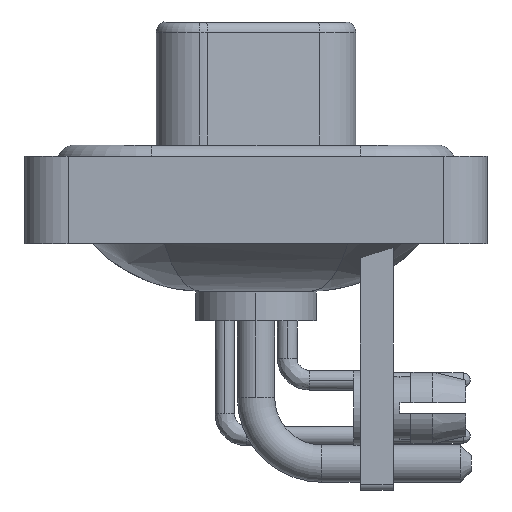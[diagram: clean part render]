
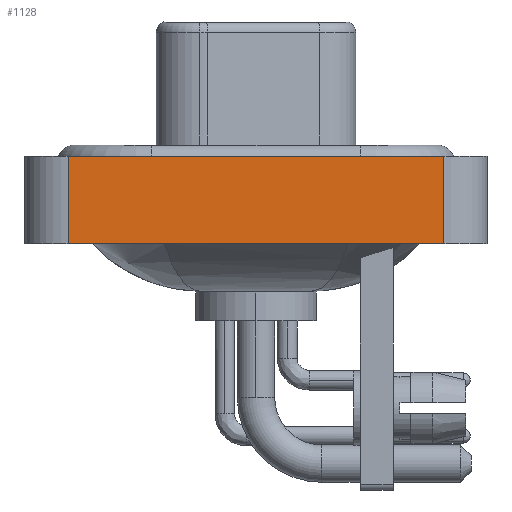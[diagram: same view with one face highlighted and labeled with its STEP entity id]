
A CAD part, left-side view. The second image highlights one B-rep face of the part: STEP entity #1128.
In plain terms, the highlighted planar face has unit normal (-1, 0, 0).
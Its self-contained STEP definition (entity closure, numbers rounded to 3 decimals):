
#1128 = ADVANCED_FACE ( 'NONE', ( #11209 ), #13248, .T. ) ;
#1898 = CARTESIAN_POINT ( 'NONE',  ( -7.3, -8.55, -3.6 ) ) ;
#1907 = DIRECTION ( 'NONE',  ( 0., -1., 0. ) ) ;
#2004 = LINE ( 'NONE', #8308, #26849 ) ;
#3120 = CARTESIAN_POINT ( 'NONE',  ( -7.3, 8.55, -3.6 ) ) ;
#3679 = VERTEX_POINT ( 'NONE', #11744 ) ;
#3937 = DIRECTION ( 'NONE',  ( 0., 0., 1. ) ) ;
#4136 = EDGE_CURVE ( 'NONE', #19035, #3679, #15676, .T. ) ;
#4199 = ORIENTED_EDGE ( 'NONE', *, *, #4136, .F. ) ;
#5425 = VERTEX_POINT ( 'NONE', #26223 ) ;
#7392 = VECTOR ( 'NONE', #19734, 1000. ) ;
#8188 = AXIS2_PLACEMENT_3D ( 'NONE', #15443, #19654, #15731 ) ;
#8308 = CARTESIAN_POINT ( 'NONE',  ( -7.3, -8.55, 0.4 ) ) ;
#8679 = VECTOR ( 'NONE', #16753, 1000. ) ;
#10782 = ORIENTED_EDGE ( 'NONE', *, *, #14921, .T. ) ;
#11209 = FACE_OUTER_BOUND ( 'NONE', #12817, .T. ) ;
#11744 = CARTESIAN_POINT ( 'NONE',  ( -7.3, 8.55, 0.4 ) ) ;
#12044 = EDGE_CURVE ( 'NONE', #19035, #5425, #12382, .T. ) ;
#12382 = LINE ( 'NONE', #1898, #8679 ) ;
#12817 = EDGE_LOOP ( 'NONE', ( #10782, #26274, #4199, #24567 ) ) ;
#13248 = PLANE ( 'NONE',  #8188 ) ;
#14921 = EDGE_CURVE ( 'NONE', #5425, #16706, #25153, .T. ) ;
#15443 = CARTESIAN_POINT ( 'NONE',  ( -7.3, -8.55, -3.6 ) ) ;
#15676 = LINE ( 'NONE', #3120, #7392 ) ;
#15731 = DIRECTION ( 'NONE',  ( 0., 0., 1. ) ) ;
#16704 = CARTESIAN_POINT ( 'NONE',  ( -7.3, -8.55, 0.4 ) ) ;
#16706 = VERTEX_POINT ( 'NONE', #16704 ) ;
#16753 = DIRECTION ( 'NONE',  ( 0., -1., 0. ) ) ;
#17656 = EDGE_CURVE ( 'NONE', #3679, #16706, #2004, .T. ) ;
#19035 = VERTEX_POINT ( 'NONE', #25343 ) ;
#19654 = DIRECTION ( 'NONE',  ( -1., 0., 0. ) ) ;
#19734 = DIRECTION ( 'NONE',  ( 0., 0., 1. ) ) ;
#22572 = CARTESIAN_POINT ( 'NONE',  ( -7.3, -8.55, -3.6 ) ) ;
#22669 = VECTOR ( 'NONE', #3937, 1000. ) ;
#24567 = ORIENTED_EDGE ( 'NONE', *, *, #12044, .T. ) ;
#25153 = LINE ( 'NONE', #22572, #22669 ) ;
#25343 = CARTESIAN_POINT ( 'NONE',  ( -7.3, 8.55, -3.6 ) ) ;
#26223 = CARTESIAN_POINT ( 'NONE',  ( -7.3, -8.55, -3.6 ) ) ;
#26274 = ORIENTED_EDGE ( 'NONE', *, *, #17656, .F. ) ;
#26849 = VECTOR ( 'NONE', #1907, 1000. ) ;
